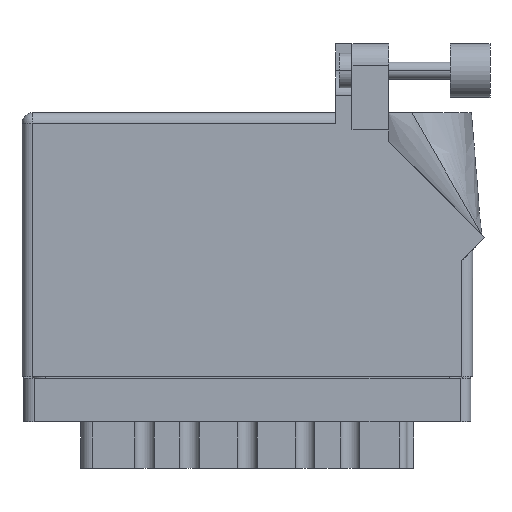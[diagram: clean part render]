
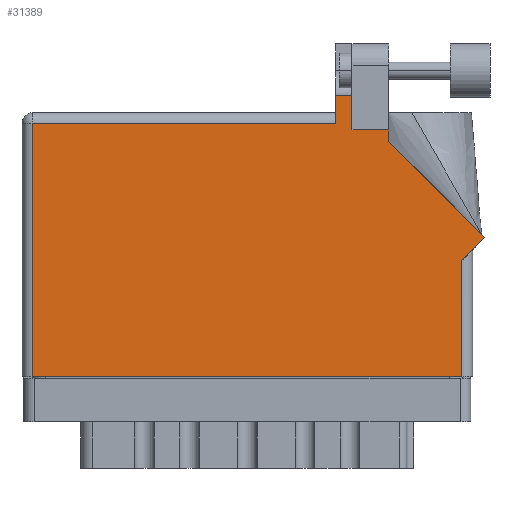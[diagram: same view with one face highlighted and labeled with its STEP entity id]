
A CAD part, front view. The second image highlights one B-rep face of the part: STEP entity #31389.
In plain terms, the highlighted face is planar.
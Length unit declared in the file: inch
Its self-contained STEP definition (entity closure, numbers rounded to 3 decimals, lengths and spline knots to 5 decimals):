
#406 = DIRECTION ( 'NONE',  ( 0.707, 0.707, 0. ) ) ;
#417 = EDGE_CURVE ( 'NONE', #51439, #7367, #53217, .T. ) ;
#721 = CARTESIAN_POINT ( 'NONE',  ( 1.819, 1.468, 0. ) ) ;
#1033 = VERTEX_POINT ( 'NONE', #5811 ) ;
#3007 = FACE_OUTER_BOUND ( 'NONE', #25639, .T. ) ;
#3163 = CARTESIAN_POINT ( 'NONE',  ( 0., 0., 0. ) ) ;
#3287 = CARTESIAN_POINT ( 'NONE',  ( 0., 1.468, 0. ) ) ;
#3994 = VERTEX_POINT ( 'NONE', #5634 ) ;
#4419 = ORIENTED_EDGE ( 'NONE', *, *, #42250, .T. ) ;
#5235 = VECTOR ( 'NONE', #35473, 39.37008 ) ;
#5634 = CARTESIAN_POINT ( 'NONE',  ( 1.913, 1.43, 0. ) ) ;
#5811 = CARTESIAN_POINT ( 'NONE',  ( 0.062, 1.468, 0. ) ) ;
#6147 = ORIENTED_EDGE ( 'NONE', *, *, #27697, .T. ) ;
#6228 = DIRECTION ( 'NONE',  ( -0.707, 0.707, 0. ) ) ;
#6371 = CARTESIAN_POINT ( 'NONE',  ( 1.913, 1.43, 0. ) ) ;
#6896 = CARTESIAN_POINT ( 'NONE',  ( 0., 1.53, 0. ) ) ;
#7367 = VERTEX_POINT ( 'NONE', #49926 ) ;
#7737 = CARTESIAN_POINT ( 'NONE',  ( 2.55, 0., 0. ) ) ;
#8975 = DIRECTION ( 'NONE',  ( 0., 1., 0. ) ) ;
#9543 = DIRECTION ( 'NONE',  ( 0., -1., 0. ) ) ;
#9989 = LINE ( 'NONE', #40726, #47749 ) ;
#10590 = VERTEX_POINT ( 'NONE', #29662 ) ;
#11040 = CARTESIAN_POINT ( 'NONE',  ( 2.24377, 1.6315, 0. ) ) ;
#11828 = ORIENTED_EDGE ( 'NONE', *, *, #45462, .T. ) ;
#12495 = CARTESIAN_POINT ( 'NONE',  ( 0.062, 0., 0. ) ) ;
#15623 = VERTEX_POINT ( 'NONE', #51007 ) ;
#17277 = ORIENTED_EDGE ( 'NONE', *, *, #25985, .T. ) ;
#17551 = VERTEX_POINT ( 'NONE', #721 ) ;
#18743 = EDGE_CURVE ( 'NONE', #15623, #17551, #40812, .T. ) ;
#20366 = ORIENTED_EDGE ( 'NONE', *, *, #22856, .T. ) ;
#20569 = ORIENTED_EDGE ( 'NONE', *, *, #417, .T. ) ;
#20951 = VECTOR ( 'NONE', #6228, 39.37008 ) ;
#21338 = CARTESIAN_POINT ( 'NONE',  ( 2.55, 0.737, 0. ) ) ;
#21432 = ORIENTED_EDGE ( 'NONE', *, *, #18743, .T. ) ;
#21820 = VERTEX_POINT ( 'NONE', #52145 ) ;
#22602 = CARTESIAN_POINT ( 'NONE',  ( 2.126, 1.43, 0. ) ) ;
#22856 = EDGE_CURVE ( 'NONE', #10590, #48296, #51140, .T. ) ;
#23618 = DIRECTION ( 'NONE',  ( 0., 0., -1. ) ) ;
#24683 = LINE ( 'NONE', #3287, #27276 ) ;
#24893 = ORIENTED_EDGE ( 'NONE', *, *, #24961, .T. ) ;
#24915 = AXIS2_PLACEMENT_3D ( 'NONE', #6896, #23618, #35634 ) ;
#24961 = EDGE_CURVE ( 'NONE', #1033, #21820, #45025, .T. ) ;
#25639 = EDGE_LOOP ( 'NONE', ( #4419, #27471, #21432, #17277, #24893, #42206, #20569, #11828, #6147, #20366, #42845 ) ) ;
#25711 = CARTESIAN_POINT ( 'NONE',  ( 1.819, 1.53, 0. ) ) ;
#25985 = EDGE_CURVE ( 'NONE', #17551, #1033, #24683, .T. ) ;
#27276 = VECTOR ( 'NONE', #48452, 39.37008 ) ;
#27345 = LINE ( 'NONE', #6371, #5235 ) ;
#27471 = ORIENTED_EDGE ( 'NONE', *, *, #34071, .T. ) ;
#27607 = PLANE ( 'NONE',  #24915 ) ;
#27697 = EDGE_CURVE ( 'NONE', #44245, #10590, #52244, .T. ) ;
#28134 = DIRECTION ( 'NONE',  ( -1., 0., 0. ) ) ;
#29392 = VECTOR ( 'NONE', #31951, 39.37008 ) ;
#29662 = CARTESIAN_POINT ( 'NONE',  ( 2.126, 1.36442, 0. ) ) ;
#30780 = CARTESIAN_POINT ( 'NONE',  ( 2.68271, 0.80771, 0. ) ) ;
#31389 = ADVANCED_FACE ( 'NONE', ( #3007 ), #27607, .F. ) ;
#31709 = VECTOR ( 'NONE', #9543, 39.37008 ) ;
#31870 = CARTESIAN_POINT ( 'NONE',  ( 1.913, 1.6315, 0. ) ) ;
#31951 = DIRECTION ( 'NONE',  ( -1., 0., 0. ) ) ;
#32006 = CARTESIAN_POINT ( 'NONE',  ( 2.68271, 0.80771, 0. ) ) ;
#32863 = LINE ( 'NONE', #38091, #45920 ) ;
#32883 = CARTESIAN_POINT ( 'NONE',  ( 2.126, 1.36442, 0. ) ) ;
#33915 = VECTOR ( 'NONE', #42148, 39.37008 ) ;
#34071 = EDGE_CURVE ( 'NONE', #38080, #15623, #37277, .T. ) ;
#34646 = LINE ( 'NONE', #3163, #45077 ) ;
#35473 = DIRECTION ( 'NONE',  ( 0., 1., 0. ) ) ;
#35634 = DIRECTION ( 'NONE',  ( -1., 0., 0. ) ) ;
#37277 = LINE ( 'NONE', #11040, #29392 ) ;
#38080 = VERTEX_POINT ( 'NONE', #31870 ) ;
#38091 = CARTESIAN_POINT ( 'NONE',  ( 2.612, 0.737, 0. ) ) ;
#38122 = VECTOR ( 'NONE', #42161, 39.37008 ) ;
#40570 = EDGE_CURVE ( 'NONE', #48296, #3994, #9989, .T. ) ;
#40726 = CARTESIAN_POINT ( 'NONE',  ( 2.126, 1.43, 0. ) ) ;
#40812 = LINE ( 'NONE', #25711, #31709 ) ;
#40819 = VECTOR ( 'NONE', #8975, 39.37008 ) ;
#41082 = EDGE_CURVE ( 'NONE', #21820, #51439, #34646, .T. ) ;
#42148 = DIRECTION ( 'NONE',  ( 0., -1., 0. ) ) ;
#42161 = DIRECTION ( 'NONE',  ( 0., 1., 0. ) ) ;
#42206 = ORIENTED_EDGE ( 'NONE', *, *, #41082, .T. ) ;
#42250 = EDGE_CURVE ( 'NONE', #3994, #38080, #27345, .T. ) ;
#42845 = ORIENTED_EDGE ( 'NONE', *, *, #40570, .T. ) ;
#44245 = VERTEX_POINT ( 'NONE', #32006 ) ;
#44495 = DIRECTION ( 'NONE',  ( 1., 0., 0. ) ) ;
#45025 = LINE ( 'NONE', #12495, #33915 ) ;
#45077 = VECTOR ( 'NONE', #44495, 39.37008 ) ;
#45462 = EDGE_CURVE ( 'NONE', #7367, #44245, #32863, .T. ) ;
#45920 = VECTOR ( 'NONE', #406, 39.37008 ) ;
#47749 = VECTOR ( 'NONE', #28134, 39.37008 ) ;
#48296 = VERTEX_POINT ( 'NONE', #22602 ) ;
#48452 = DIRECTION ( 'NONE',  ( -1., 0., 0. ) ) ;
#49926 = CARTESIAN_POINT ( 'NONE',  ( 2.55, 0.675, 0. ) ) ;
#51007 = CARTESIAN_POINT ( 'NONE',  ( 1.819, 1.6315, 0. ) ) ;
#51140 = LINE ( 'NONE', #32883, #38122 ) ;
#51439 = VERTEX_POINT ( 'NONE', #7737 ) ;
#52145 = CARTESIAN_POINT ( 'NONE',  ( 0.062, 0., 0. ) ) ;
#52244 = LINE ( 'NONE', #30780, #20951 ) ;
#53217 = LINE ( 'NONE', #21338, #40819 ) ;
